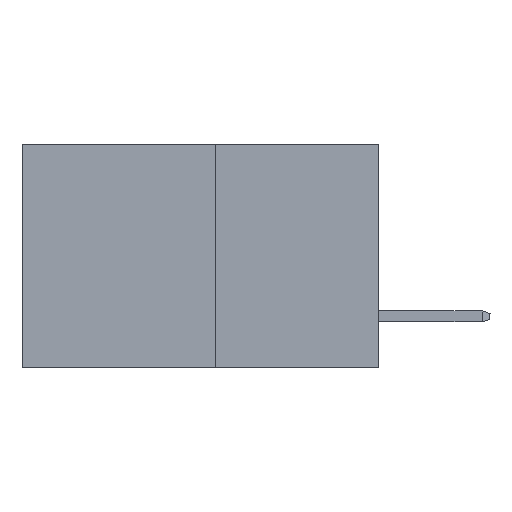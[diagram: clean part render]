
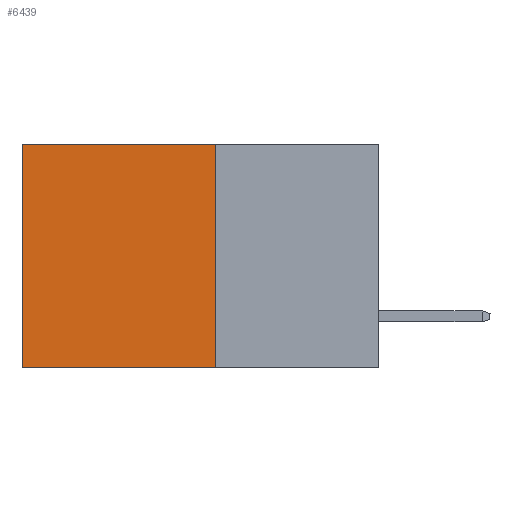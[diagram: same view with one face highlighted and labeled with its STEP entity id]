
A CAD part, left-side view. The second image highlights one B-rep face of the part: STEP entity #6439.
In plain terms, the highlighted planar face has unit normal (-1, 0, 0).
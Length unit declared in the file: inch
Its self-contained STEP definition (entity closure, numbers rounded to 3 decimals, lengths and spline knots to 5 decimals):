
#95 = ORIENTED_EDGE ( 'NONE', *, *, #2981, .T. ) ;
#333 = CARTESIAN_POINT ( 'NONE',  ( 0.277, 0.27, -0.37 ) ) ;
#388 = DIRECTION ( 'NONE',  ( 0., 0., -1. ) ) ;
#400 = DIRECTION ( 'NONE',  ( 1., 0., 0. ) ) ;
#508 = VECTOR ( 'NONE', #8537, 39.37008 ) ;
#519 = PLANE ( 'NONE',  #8895 ) ;
#601 = CARTESIAN_POINT ( 'NONE',  ( 0.277, 0.27, -0.37 ) ) ;
#707 = VERTEX_POINT ( 'NONE', #3681 ) ;
#1671 = VERTEX_POINT ( 'NONE', #333 ) ;
#1826 = VERTEX_POINT ( 'NONE', #1900 ) ;
#1865 = VECTOR ( 'NONE', #5317, 39.37008 ) ;
#1900 = CARTESIAN_POINT ( 'NONE',  ( 0.277, 0.59, -0.37 ) ) ;
#2229 = LINE ( 'NONE', #3979, #7980 ) ;
#2981 = EDGE_CURVE ( 'NONE', #707, #5836, #2229, .T. ) ;
#3681 = CARTESIAN_POINT ( 'NONE',  ( 0.277, 0.27, 0. ) ) ;
#3748 = LINE ( 'NONE', #9547, #1865 ) ;
#3979 = CARTESIAN_POINT ( 'NONE',  ( 0.277, 0.27, 0. ) ) ;
#4060 = VECTOR ( 'NONE', #8832, 39.37008 ) ;
#4736 = LINE ( 'NONE', #8548, #508 ) ;
#5213 = EDGE_CURVE ( 'NONE', #707, #1671, #7939, .T. ) ;
#5317 = DIRECTION ( 'NONE',  ( 0., 1., 0. ) ) ;
#5782 = CARTESIAN_POINT ( 'NONE',  ( 0.277, 0.27, -0.37 ) ) ;
#5836 = VERTEX_POINT ( 'NONE', #6475 ) ;
#6439 = ADVANCED_FACE ( 'NONE', ( #8590 ), #519, .F. ) ;
#6475 = CARTESIAN_POINT ( 'NONE',  ( 0.277, 0.59, 0. ) ) ;
#7085 = ORIENTED_EDGE ( 'NONE', *, *, #5213, .F. ) ;
#7230 = EDGE_CURVE ( 'NONE', #5836, #1826, #4736, .T. ) ;
#7777 = EDGE_LOOP ( 'NONE', ( #7940, #8730, #7085, #95 ) ) ;
#7939 = LINE ( 'NONE', #5782, #4060 ) ;
#7940 = ORIENTED_EDGE ( 'NONE', *, *, #7230, .T. ) ;
#7980 = VECTOR ( 'NONE', #9007, 39.37008 ) ;
#8537 = DIRECTION ( 'NONE',  ( 0., 0., -1. ) ) ;
#8548 = CARTESIAN_POINT ( 'NONE',  ( 0.277, 0.59, -0.37 ) ) ;
#8590 = FACE_OUTER_BOUND ( 'NONE', #7777, .T. ) ;
#8730 = ORIENTED_EDGE ( 'NONE', *, *, #9614, .F. ) ;
#8832 = DIRECTION ( 'NONE',  ( 0., 0., -1. ) ) ;
#8895 = AXIS2_PLACEMENT_3D ( 'NONE', #601, #400, #388 ) ;
#9007 = DIRECTION ( 'NONE',  ( 0., 1., 0. ) ) ;
#9547 = CARTESIAN_POINT ( 'NONE',  ( 0.277, 0.27, -0.37 ) ) ;
#9614 = EDGE_CURVE ( 'NONE', #1671, #1826, #3748, .T. ) ;
